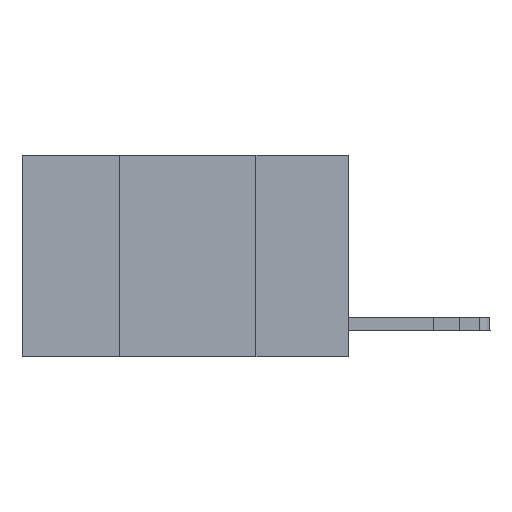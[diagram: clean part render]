
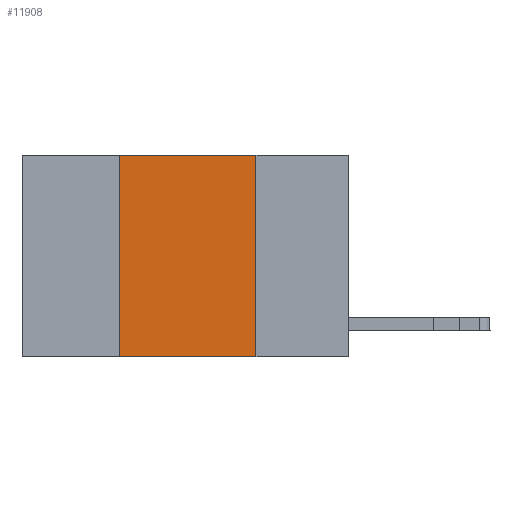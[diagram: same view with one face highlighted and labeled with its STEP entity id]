
A CAD part, left-side view. The second image highlights one B-rep face of the part: STEP entity #11908.
In plain terms, the highlighted planar face has unit normal (-1, 0, 0).
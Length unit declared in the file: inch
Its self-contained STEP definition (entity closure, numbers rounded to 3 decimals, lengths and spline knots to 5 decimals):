
#868 = CARTESIAN_POINT ( 'NONE',  ( 0., 0.6, 0. ) ) ;
#1888 = VECTOR ( 'NONE', #11789, 39.37008 ) ;
#3148 = CARTESIAN_POINT ( 'NONE',  ( 0., 0.6, 0. ) ) ;
#3431 = CARTESIAN_POINT ( 'NONE',  ( 0., 0.42, 0. ) ) ;
#4201 = ORIENTED_EDGE ( 'NONE', *, *, #10430, .F. ) ;
#6535 = EDGE_CURVE ( 'NONE', #19280, #11973, #16523, .T. ) ;
#6668 = EDGE_LOOP ( 'NONE', ( #4201, #22003, #16299, #22567 ) ) ;
#6866 = DIRECTION ( 'NONE',  ( 0., 0., -1. ) ) ;
#7315 = CARTESIAN_POINT ( 'NONE',  ( 0., 0.17, 0. ) ) ;
#7344 = CARTESIAN_POINT ( 'NONE',  ( 0., 0.42, 0. ) ) ;
#8446 = CARTESIAN_POINT ( 'NONE',  ( 0., 0.42, -0.37 ) ) ;
#9203 = DIRECTION ( 'NONE',  ( 0., 0., -1. ) ) ;
#10430 = EDGE_CURVE ( 'NONE', #15718, #11973, #14673, .T. ) ;
#11418 = CARTESIAN_POINT ( 'NONE',  ( 0., 0.17, -0.37 ) ) ;
#11789 = DIRECTION ( 'NONE',  ( 0., -1., 0. ) ) ;
#11794 = DIRECTION ( 'NONE',  ( 0., 0., 1. ) ) ;
#11908 = ADVANCED_FACE ( 'NONE', ( #13317 ), #19612, .F. ) ;
#11973 = VERTEX_POINT ( 'NONE', #11418 ) ;
#13208 = AXIS2_PLACEMENT_3D ( 'NONE', #868, #15639, #9203 ) ;
#13317 = FACE_OUTER_BOUND ( 'NONE', #6668, .T. ) ;
#13748 = VECTOR ( 'NONE', #11794, 39.37008 ) ;
#13820 = DIRECTION ( 'NONE',  ( 0., -1., 0. ) ) ;
#14673 = LINE ( 'NONE', #15073, #17760 ) ;
#15073 = CARTESIAN_POINT ( 'NONE',  ( 0., 0.17, 0. ) ) ;
#15201 = VERTEX_POINT ( 'NONE', #7344 ) ;
#15639 = DIRECTION ( 'NONE',  ( 1., 0., 0. ) ) ;
#15718 = VERTEX_POINT ( 'NONE', #7315 ) ;
#16022 = EDGE_CURVE ( 'NONE', #15201, #15718, #22169, .T. ) ;
#16299 = ORIENTED_EDGE ( 'NONE', *, *, #20425, .F. ) ;
#16523 = LINE ( 'NONE', #26786, #1888 ) ;
#17760 = VECTOR ( 'NONE', #6866, 39.37008 ) ;
#17946 = LINE ( 'NONE', #3431, #13748 ) ;
#19280 = VERTEX_POINT ( 'NONE', #8446 ) ;
#19612 = PLANE ( 'NONE',  #13208 ) ;
#20425 = EDGE_CURVE ( 'NONE', #19280, #15201, #17946, .T. ) ;
#22003 = ORIENTED_EDGE ( 'NONE', *, *, #16022, .F. ) ;
#22169 = LINE ( 'NONE', #3148, #25868 ) ;
#22567 = ORIENTED_EDGE ( 'NONE', *, *, #6535, .T. ) ;
#25868 = VECTOR ( 'NONE', #13820, 39.37008 ) ;
#26786 = CARTESIAN_POINT ( 'NONE',  ( 0., 0.6, -0.37 ) ) ;
